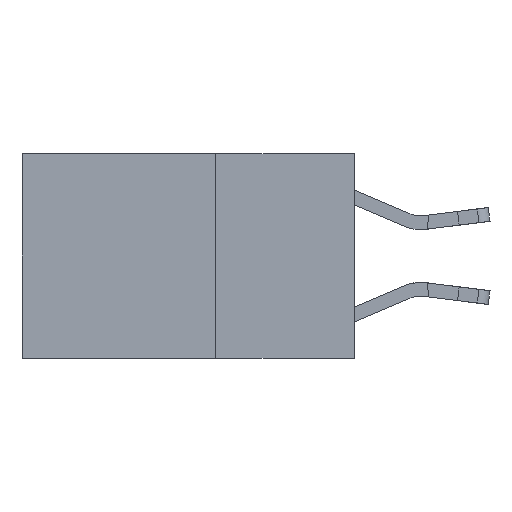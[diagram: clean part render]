
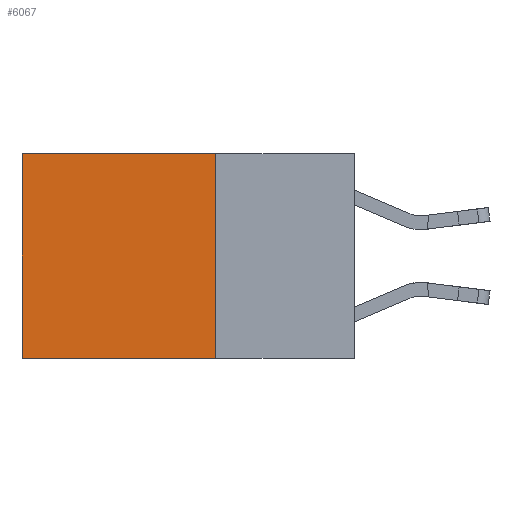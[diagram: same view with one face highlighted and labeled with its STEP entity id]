
A CAD part, left-side view. The second image highlights one B-rep face of the part: STEP entity #6067.
In plain terms, the highlighted planar face has unit normal (-1, 0, 0).
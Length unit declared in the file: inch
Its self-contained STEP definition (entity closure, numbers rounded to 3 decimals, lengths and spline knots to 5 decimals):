
#1750 = AXIS2_PLACEMENT_3D ( 'NONE', #4784, #12396, #19979 ) ;
#1884 = EDGE_CURVE ( 'NONE', #18950, #19622, #3788, .T. ) ;
#2509 = CARTESIAN_POINT ( 'NONE',  ( 0.2625, 0.25, 0. ) ) ;
#2631 = LINE ( 'NONE', #2509, #8399 ) ;
#3145 = ORIENTED_EDGE ( 'NONE', *, *, #22032, .T. ) ;
#3693 = EDGE_LOOP ( 'NONE', ( #5543, #4510, #22573, #3145 ) ) ;
#3788 = LINE ( 'NONE', #13390, #8758 ) ;
#4182 = CARTESIAN_POINT ( 'NONE',  ( 0.2625, 0.6, 0. ) ) ;
#4461 = VERTEX_POINT ( 'NONE', #4182 ) ;
#4510 = ORIENTED_EDGE ( 'NONE', *, *, #20833, .F. ) ;
#4784 = CARTESIAN_POINT ( 'NONE',  ( 0.2625, 0.25, 0. ) ) ;
#5543 = ORIENTED_EDGE ( 'NONE', *, *, #22673, .T. ) ;
#6067 = ADVANCED_FACE ( 'NONE', ( #10636 ), #21831, .F. ) ;
#6403 = DIRECTION ( 'NONE',  ( 0., 1., 0. ) ) ;
#8399 = VECTOR ( 'NONE', #6403, 39.37008 ) ;
#8758 = VECTOR ( 'NONE', #11011, 39.37008 ) ;
#9455 = CARTESIAN_POINT ( 'NONE',  ( 0.2625, 0.6, 0. ) ) ;
#10636 = FACE_OUTER_BOUND ( 'NONE', #3693, .T. ) ;
#11011 = DIRECTION ( 'NONE',  ( 0., 0., -1. ) ) ;
#11434 = LINE ( 'NONE', #9455, #15970 ) ;
#12396 = DIRECTION ( 'NONE',  ( 1., 0., 0. ) ) ;
#13390 = CARTESIAN_POINT ( 'NONE',  ( 0.2625, 0.25, 0. ) ) ;
#15188 = DIRECTION ( 'NONE',  ( 0., 0., -1. ) ) ;
#15565 = VECTOR ( 'NONE', #16740, 39.37008 ) ;
#15970 = VECTOR ( 'NONE', #15188, 39.37008 ) ;
#16676 = CARTESIAN_POINT ( 'NONE',  ( 0.2625, 0.25, -0.37 ) ) ;
#16740 = DIRECTION ( 'NONE',  ( 0., 1., 0. ) ) ;
#18387 = CARTESIAN_POINT ( 'NONE',  ( 0.2625, 0.6, -0.37 ) ) ;
#18600 = LINE ( 'NONE', #22689, #15565 ) ;
#18950 = VERTEX_POINT ( 'NONE', #19222 ) ;
#19222 = CARTESIAN_POINT ( 'NONE',  ( 0.2625, 0.25, 0. ) ) ;
#19622 = VERTEX_POINT ( 'NONE', #16676 ) ;
#19979 = DIRECTION ( 'NONE',  ( 0., 0., -1. ) ) ;
#20833 = EDGE_CURVE ( 'NONE', #19622, #24442, #18600, .T. ) ;
#21831 = PLANE ( 'NONE',  #1750 ) ;
#22032 = EDGE_CURVE ( 'NONE', #18950, #4461, #2631, .T. ) ;
#22573 = ORIENTED_EDGE ( 'NONE', *, *, #1884, .F. ) ;
#22673 = EDGE_CURVE ( 'NONE', #4461, #24442, #11434, .T. ) ;
#22689 = CARTESIAN_POINT ( 'NONE',  ( 0.2625, 0.25, -0.37 ) ) ;
#24442 = VERTEX_POINT ( 'NONE', #18387 ) ;
